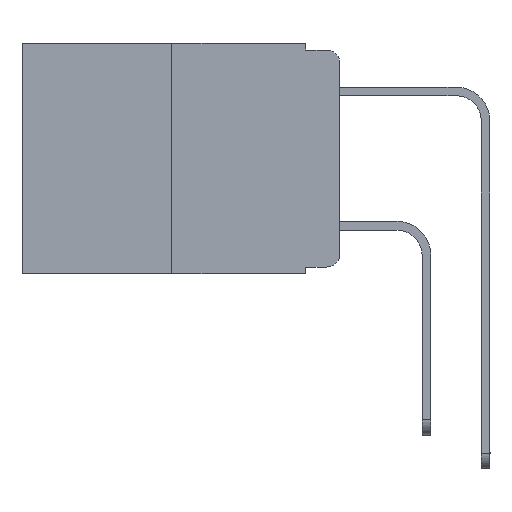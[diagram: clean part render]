
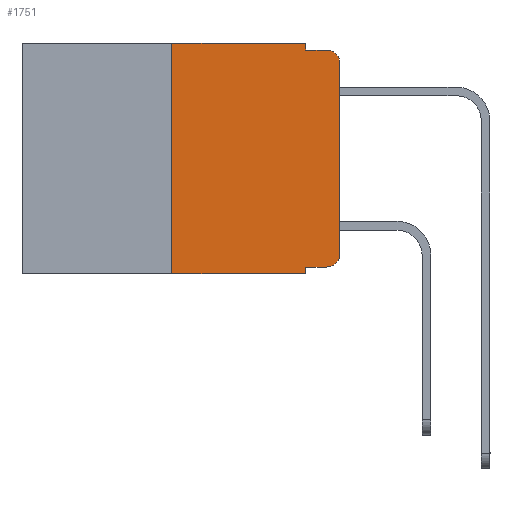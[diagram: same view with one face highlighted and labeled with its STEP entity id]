
A CAD part, left-side view. The second image highlights one B-rep face of the part: STEP entity #1751.
In plain terms, the highlighted planar face has unit normal (-1, 0, 0).
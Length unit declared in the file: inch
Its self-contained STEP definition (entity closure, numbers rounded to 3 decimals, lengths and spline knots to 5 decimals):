
#62 = CARTESIAN_POINT ( 'NONE',  ( 0., 0.051, -0.01 ) ) ;
#624 = FACE_OUTER_BOUND ( 'NONE', #4988, .T. ) ;
#880 = DIRECTION ( 'NONE',  ( 0., 0., -1. ) ) ;
#1310 = EDGE_CURVE ( 'NONE', #14167, #2532, #1856, .T. ) ;
#1380 = EDGE_CURVE ( 'NONE', #13694, #12689, #9287, .T. ) ;
#1568 = ORIENTED_EDGE ( 'NONE', *, *, #6022, .T. ) ;
#1665 = EDGE_CURVE ( 'NONE', #9338, #14167, #11076, .T. ) ;
#1751 = ADVANCED_FACE ( 'NONE', ( #624 ), #11154, .F. ) ;
#1797 = CARTESIAN_POINT ( 'NONE',  ( 0., 0.25, -0.343 ) ) ;
#1820 = ORIENTED_EDGE ( 'NONE', *, *, #1310, .F. ) ;
#1856 = LINE ( 'NONE', #5311, #10559 ) ;
#2287 = CARTESIAN_POINT ( 'NONE',  ( 0., 0.051, 0. ) ) ;
#2359 = CARTESIAN_POINT ( 'NONE',  ( 0., 0.25, 0. ) ) ;
#2532 = VERTEX_POINT ( 'NONE', #62 ) ;
#2917 = DIRECTION ( 'NONE',  ( 0., -1., 0. ) ) ;
#3435 = ORIENTED_EDGE ( 'NONE', *, *, #6777, .T. ) ;
#3554 = CARTESIAN_POINT ( 'NONE',  ( 0., 0.051, -0.01 ) ) ;
#3907 = ORIENTED_EDGE ( 'NONE', *, *, #1380, .T. ) ;
#4313 = DIRECTION ( 'NONE',  ( 0., 0., -1. ) ) ;
#4353 = LINE ( 'NONE', #12801, #6581 ) ;
#4362 = CARTESIAN_POINT ( 'NONE',  ( 0., 0., -0.03 ) ) ;
#4664 = DIRECTION ( 'NONE',  ( 0., -1., 0. ) ) ;
#4865 = CIRCLE ( 'NONE', #10698, 0.02 ) ;
#4891 = CARTESIAN_POINT ( 'NONE',  ( 0., 0., -0.313 ) ) ;
#4910 = VECTOR ( 'NONE', #8871, 39.37008 ) ;
#4988 = EDGE_LOOP ( 'NONE', ( #1568, #11416, #14044, #1820, #9557, #14089, #3907, #13963, #5318, #3435 ) ) ;
#5004 = CARTESIAN_POINT ( 'NONE',  ( 0., 0.051, -0.333 ) ) ;
#5150 = CARTESIAN_POINT ( 'NONE',  ( 0., 0.02, -0.03 ) ) ;
#5311 = CARTESIAN_POINT ( 'NONE',  ( 0., 0.051, 0. ) ) ;
#5318 = ORIENTED_EDGE ( 'NONE', *, *, #9404, .T. ) ;
#5689 = VECTOR ( 'NONE', #12691, 39.37008 ) ;
#5893 = VERTEX_POINT ( 'NONE', #4362 ) ;
#6022 = EDGE_CURVE ( 'NONE', #6566, #5893, #11438, .T. ) ;
#6391 = CARTESIAN_POINT ( 'NONE',  ( 0., 0.473, 0. ) ) ;
#6566 = VERTEX_POINT ( 'NONE', #4891 ) ;
#6581 = VECTOR ( 'NONE', #4664, 39.37008 ) ;
#6648 = CARTESIAN_POINT ( 'NONE',  ( 0., 0.02, -0.313 ) ) ;
#6757 = DIRECTION ( 'NONE',  ( 0., 0., 1. ) ) ;
#6777 = EDGE_CURVE ( 'NONE', #14387, #6566, #4865, .T. ) ;
#6984 = LINE ( 'NONE', #2359, #10439 ) ;
#6994 = CARTESIAN_POINT ( 'NONE',  ( 0., 0.473, -0.343 ) ) ;
#8195 = VECTOR ( 'NONE', #10160, 39.37008 ) ;
#8287 = CARTESIAN_POINT ( 'NONE',  ( 0., 0.02, -0.333 ) ) ;
#8813 = VECTOR ( 'NONE', #12846, 39.37008 ) ;
#8871 = DIRECTION ( 'NONE',  ( 0., 0., -1. ) ) ;
#8938 = CARTESIAN_POINT ( 'NONE',  ( 0., 0.051, 0. ) ) ;
#8960 = CARTESIAN_POINT ( 'NONE',  ( 0., 0., 0. ) ) ;
#8969 = EDGE_CURVE ( 'NONE', #13694, #9338, #6984, .T. ) ;
#9088 = EDGE_CURVE ( 'NONE', #5893, #9351, #10935, .T. ) ;
#9226 = LINE ( 'NONE', #3554, #8813 ) ;
#9287 = LINE ( 'NONE', #6994, #5689 ) ;
#9338 = VERTEX_POINT ( 'NONE', #13781 ) ;
#9351 = VERTEX_POINT ( 'NONE', #11577 ) ;
#9404 = EDGE_CURVE ( 'NONE', #14331, #14387, #4353, .T. ) ;
#9557 = ORIENTED_EDGE ( 'NONE', *, *, #1665, .F. ) ;
#10065 = AXIS2_PLACEMENT_3D ( 'NONE', #12080, #10936, #14659 ) ;
#10141 = LINE ( 'NONE', #8938, #4910 ) ;
#10160 = DIRECTION ( 'NONE',  ( 0., 0., 1. ) ) ;
#10439 = VECTOR ( 'NONE', #6757, 39.37008 ) ;
#10559 = VECTOR ( 'NONE', #4313, 39.37008 ) ;
#10698 = AXIS2_PLACEMENT_3D ( 'NONE', #6648, #12490, #880 ) ;
#10851 = DIRECTION ( 'NONE',  ( -1., 0., 0. ) ) ;
#10897 = EDGE_CURVE ( 'NONE', #14331, #12689, #10141, .T. ) ;
#10935 = CIRCLE ( 'NONE', #12151, 0.02 ) ;
#10936 = DIRECTION ( 'NONE',  ( 1., 0., 0. ) ) ;
#11076 = LINE ( 'NONE', #6391, #14695 ) ;
#11154 = PLANE ( 'NONE',  #10065 ) ;
#11416 = ORIENTED_EDGE ( 'NONE', *, *, #9088, .T. ) ;
#11438 = LINE ( 'NONE', #8960, #8195 ) ;
#11577 = CARTESIAN_POINT ( 'NONE',  ( 0., 0.02, -0.01 ) ) ;
#11939 = CARTESIAN_POINT ( 'NONE',  ( 0., 0.051, -0.343 ) ) ;
#12080 = CARTESIAN_POINT ( 'NONE',  ( 0., 0.473, 0. ) ) ;
#12151 = AXIS2_PLACEMENT_3D ( 'NONE', #5150, #10851, #12982 ) ;
#12490 = DIRECTION ( 'NONE',  ( -1., 0., 0. ) ) ;
#12689 = VERTEX_POINT ( 'NONE', #11939 ) ;
#12691 = DIRECTION ( 'NONE',  ( 0., -1., 0. ) ) ;
#12801 = CARTESIAN_POINT ( 'NONE',  ( 0., 0.051, -0.333 ) ) ;
#12846 = DIRECTION ( 'NONE',  ( 0., -1., 0. ) ) ;
#12982 = DIRECTION ( 'NONE',  ( 0., 0., -1. ) ) ;
#13694 = VERTEX_POINT ( 'NONE', #1797 ) ;
#13781 = CARTESIAN_POINT ( 'NONE',  ( 0., 0.25, 0. ) ) ;
#13963 = ORIENTED_EDGE ( 'NONE', *, *, #10897, .F. ) ;
#14044 = ORIENTED_EDGE ( 'NONE', *, *, #15044, .F. ) ;
#14089 = ORIENTED_EDGE ( 'NONE', *, *, #8969, .F. ) ;
#14167 = VERTEX_POINT ( 'NONE', #2287 ) ;
#14331 = VERTEX_POINT ( 'NONE', #5004 ) ;
#14387 = VERTEX_POINT ( 'NONE', #8287 ) ;
#14659 = DIRECTION ( 'NONE',  ( 0., 0., -1. ) ) ;
#14695 = VECTOR ( 'NONE', #2917, 39.37008 ) ;
#15044 = EDGE_CURVE ( 'NONE', #2532, #9351, #9226, .T. ) ;
